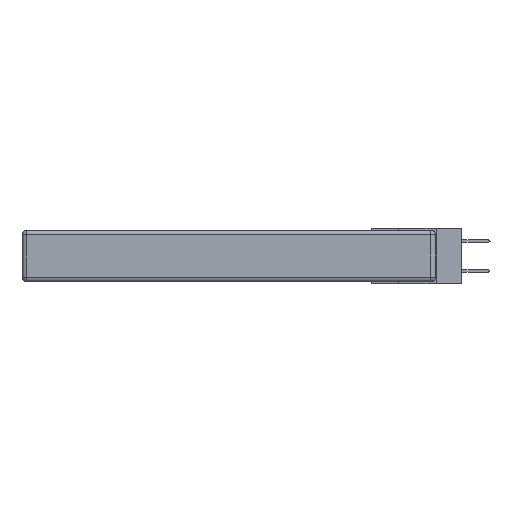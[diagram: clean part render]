
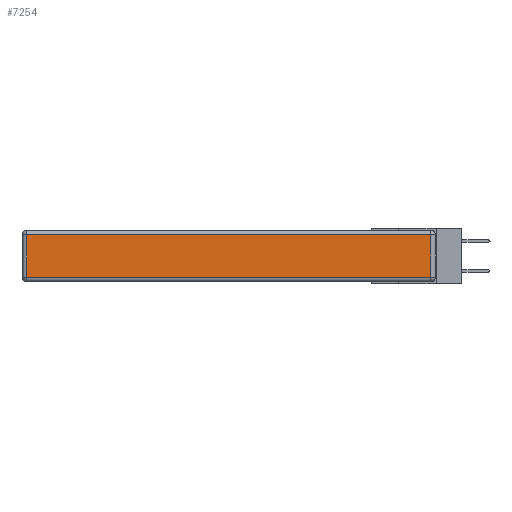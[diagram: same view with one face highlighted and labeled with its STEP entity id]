
A CAD part, left-side view. The second image highlights one B-rep face of the part: STEP entity #7254.
In plain terms, the highlighted planar face has unit normal (-1, 0, 0).
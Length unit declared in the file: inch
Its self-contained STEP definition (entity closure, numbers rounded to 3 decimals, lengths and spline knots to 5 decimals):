
#769 = VECTOR ( 'NONE', #10039, 39.37008 ) ;
#1565 = VECTOR ( 'NONE', #16317, 39.37008 ) ;
#1878 = CARTESIAN_POINT ( 'NONE',  ( 0., 2.72, -0.313 ) ) ;
#4835 = EDGE_CURVE ( 'NONE', #16739, #18643, #12557, .T. ) ;
#5962 = DIRECTION ( 'NONE',  ( 0., 0., -1. ) ) ;
#6201 = PLANE ( 'NONE',  #27561 ) ;
#6958 = ORIENTED_EDGE ( 'NONE', *, *, #17266, .T. ) ;
#7254 = ADVANCED_FACE ( 'NONE', ( #23065 ), #6201, .T. ) ;
#7663 = LINE ( 'NONE', #8133, #9370 ) ;
#8133 = CARTESIAN_POINT ( 'NONE',  ( 0., 2.75, -0.03 ) ) ;
#8161 = ORIENTED_EDGE ( 'NONE', *, *, #22447, .T. ) ;
#8682 = VERTEX_POINT ( 'NONE', #1878 ) ;
#9370 = VECTOR ( 'NONE', #20741, 39.37008 ) ;
#10039 = DIRECTION ( 'NONE',  ( 0., -1., 0. ) ) ;
#10914 = CARTESIAN_POINT ( 'NONE',  ( 0., 2.72, -0.343 ) ) ;
#12557 = LINE ( 'NONE', #30412, #1565 ) ;
#12591 = CARTESIAN_POINT ( 'NONE',  ( 0., 0.03, -0.313 ) ) ;
#13042 = DIRECTION ( 'NONE',  ( -1., 0., 0. ) ) ;
#13862 = ORIENTED_EDGE ( 'NONE', *, *, #4835, .T. ) ;
#15193 = EDGE_LOOP ( 'NONE', ( #25136, #13862, #8161, #6958 ) ) ;
#15637 = LINE ( 'NONE', #10914, #29270 ) ;
#15857 = VERTEX_POINT ( 'NONE', #19782 ) ;
#16317 = DIRECTION ( 'NONE',  ( 0., 0., 1. ) ) ;
#16739 = VERTEX_POINT ( 'NONE', #12591 ) ;
#17266 = EDGE_CURVE ( 'NONE', #15857, #8682, #15637, .T. ) ;
#18643 = VERTEX_POINT ( 'NONE', #30307 ) ;
#19469 = LINE ( 'NONE', #24105, #769 ) ;
#19782 = CARTESIAN_POINT ( 'NONE',  ( 0., 2.72, -0.03 ) ) ;
#20741 = DIRECTION ( 'NONE',  ( 0., 1., 0. ) ) ;
#22168 = DIRECTION ( 'NONE',  ( 0., 0., 1. ) ) ;
#22447 = EDGE_CURVE ( 'NONE', #18643, #15857, #7663, .T. ) ;
#23065 = FACE_OUTER_BOUND ( 'NONE', #15193, .T. ) ;
#24105 = CARTESIAN_POINT ( 'NONE',  ( 0., 0., -0.313 ) ) ;
#25136 = ORIENTED_EDGE ( 'NONE', *, *, #28879, .T. ) ;
#25504 = CARTESIAN_POINT ( 'NONE',  ( 0., 0., -0.343 ) ) ;
#27561 = AXIS2_PLACEMENT_3D ( 'NONE', #25504, #13042, #22168 ) ;
#28879 = EDGE_CURVE ( 'NONE', #8682, #16739, #19469, .T. ) ;
#29270 = VECTOR ( 'NONE', #5962, 39.37008 ) ;
#30307 = CARTESIAN_POINT ( 'NONE',  ( 0., 0.03, -0.03 ) ) ;
#30412 = CARTESIAN_POINT ( 'NONE',  ( 0., 0.03, -0.343 ) ) ;
